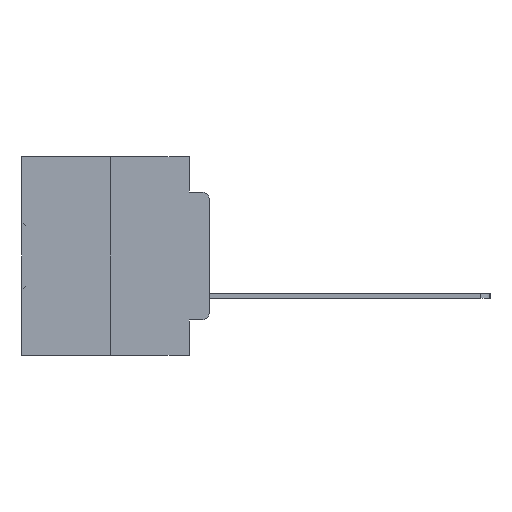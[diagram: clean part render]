
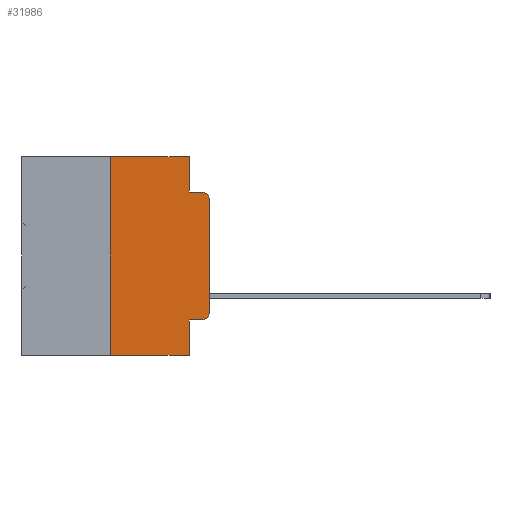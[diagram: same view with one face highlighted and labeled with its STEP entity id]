
A CAD part, left-side view. The second image highlights one B-rep face of the part: STEP entity #31986.
In plain terms, the highlighted planar face has unit normal (-1, 0, 0).
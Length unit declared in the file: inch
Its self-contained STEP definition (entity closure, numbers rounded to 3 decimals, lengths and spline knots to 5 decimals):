
#34 = CARTESIAN_POINT ( 'NONE',  ( 0., 0.051, -0.0885 ) ) ;
#468 = CARTESIAN_POINT ( 'NONE',  ( 0., 0.051, -0.5 ) ) ;
#720 = CARTESIAN_POINT ( 'NONE',  ( 0., 0.051, 0. ) ) ;
#902 = CARTESIAN_POINT ( 'NONE',  ( 0., 0.051, -0.4115 ) ) ;
#982 = CARTESIAN_POINT ( 'NONE',  ( 0., 0., -0.1085 ) ) ;
#1064 = VECTOR ( 'NONE', #9573, 39.37008 ) ;
#1065 = VERTEX_POINT ( 'NONE', #982 ) ;
#1496 = VERTEX_POINT ( 'NONE', #468 ) ;
#1793 = FACE_OUTER_BOUND ( 'NONE', #23797, .T. ) ;
#3012 = EDGE_CURVE ( 'NONE', #28477, #24583, #29889, .T. ) ;
#3042 = AXIS2_PLACEMENT_3D ( 'NONE', #6347, #25291, #9121 ) ;
#3171 = DIRECTION ( 'NONE',  ( 0., 0., 1. ) ) ;
#3943 = VECTOR ( 'NONE', #19839, 39.37008 ) ;
#4041 = DIRECTION ( 'NONE',  ( 0., -1., 0. ) ) ;
#4049 = VECTOR ( 'NONE', #10755, 39.37008 ) ;
#4893 = EDGE_CURVE ( 'NONE', #28477, #1496, #25623, .T. ) ;
#4903 = ORIENTED_EDGE ( 'NONE', *, *, #6758, .F. ) ;
#6218 = ORIENTED_EDGE ( 'NONE', *, *, #30897, .T. ) ;
#6347 = CARTESIAN_POINT ( 'NONE',  ( 0., 0.02, -0.1085 ) ) ;
#6378 = DIRECTION ( 'NONE',  ( -1., 0., 0. ) ) ;
#6604 = CARTESIAN_POINT ( 'NONE',  ( 0., 0.051, -0.0885 ) ) ;
#6731 = CARTESIAN_POINT ( 'NONE',  ( 0., 0.473, 0. ) ) ;
#6758 = EDGE_CURVE ( 'NONE', #26242, #31788, #13685, .T. ) ;
#7073 = VECTOR ( 'NONE', #21686, 39.37008 ) ;
#7951 = CARTESIAN_POINT ( 'NONE',  ( 0., 0.02, -0.4115 ) ) ;
#8803 = CIRCLE ( 'NONE', #24824, 0.02 ) ;
#8840 = LINE ( 'NONE', #6731, #29477 ) ;
#9121 = DIRECTION ( 'NONE',  ( 0., 0., -1. ) ) ;
#9237 = ORIENTED_EDGE ( 'NONE', *, *, #19950, .T. ) ;
#9573 = DIRECTION ( 'NONE',  ( 0., -1., 0. ) ) ;
#9653 = ORIENTED_EDGE ( 'NONE', *, *, #14054, .F. ) ;
#10421 = CARTESIAN_POINT ( 'NONE',  ( 0., 0.051, 0. ) ) ;
#10579 = CARTESIAN_POINT ( 'NONE',  ( 0., 0.25, -0.5 ) ) ;
#10755 = DIRECTION ( 'NONE',  ( 0., -1., 0. ) ) ;
#11082 = DIRECTION ( 'NONE',  ( 1., 0., 0. ) ) ;
#11519 = VERTEX_POINT ( 'NONE', #20777 ) ;
#11705 = DIRECTION ( 'NONE',  ( 0., 0., 1. ) ) ;
#12249 = EDGE_CURVE ( 'NONE', #25033, #15721, #30239, .T. ) ;
#13484 = LINE ( 'NONE', #6604, #18943 ) ;
#13685 = LINE ( 'NONE', #27848, #32511 ) ;
#14054 = EDGE_CURVE ( 'NONE', #15721, #17731, #13484, .T. ) ;
#15134 = ORIENTED_EDGE ( 'NONE', *, *, #15868, .T. ) ;
#15721 = VERTEX_POINT ( 'NONE', #34 ) ;
#15868 = EDGE_CURVE ( 'NONE', #1065, #17731, #16267, .T. ) ;
#16267 = CIRCLE ( 'NONE', #3042, 0.02 ) ;
#17731 = VERTEX_POINT ( 'NONE', #29797 ) ;
#18111 = ORIENTED_EDGE ( 'NONE', *, *, #4893, .F. ) ;
#18943 = VECTOR ( 'NONE', #28223, 39.37008 ) ;
#19476 = EDGE_CURVE ( 'NONE', #11519, #1065, #26607, .T. ) ;
#19839 = DIRECTION ( 'NONE',  ( 0., 0., -1. ) ) ;
#19950 = EDGE_CURVE ( 'NONE', #26242, #1496, #32732, .T. ) ;
#20318 = CARTESIAN_POINT ( 'NONE',  ( 0., 0.051, -0.4115 ) ) ;
#20777 = CARTESIAN_POINT ( 'NONE',  ( 0., 0., -0.3915 ) ) ;
#20922 = CARTESIAN_POINT ( 'NONE',  ( 0., 0.25, 0. ) ) ;
#21392 = CARTESIAN_POINT ( 'NONE',  ( 0., 0.473, -0.5 ) ) ;
#21480 = ORIENTED_EDGE ( 'NONE', *, *, #19476, .T. ) ;
#21686 = DIRECTION ( 'NONE',  ( 0., 0., -1. ) ) ;
#22640 = CARTESIAN_POINT ( 'NONE',  ( 0., 0.02, -0.3915 ) ) ;
#23797 = EDGE_LOOP ( 'NONE', ( #21480, #15134, #9653, #31063, #25699, #4903, #9237, #18111, #32322, #6218 ) ) ;
#24556 = CARTESIAN_POINT ( 'NONE',  ( 0., 0.473, 0. ) ) ;
#24583 = VERTEX_POINT ( 'NONE', #7951 ) ;
#24824 = AXIS2_PLACEMENT_3D ( 'NONE', #22640, #6378, #25323 ) ;
#25033 = VERTEX_POINT ( 'NONE', #10421 ) ;
#25291 = DIRECTION ( 'NONE',  ( -1., 0., 0. ) ) ;
#25323 = DIRECTION ( 'NONE',  ( 0., 0., -1. ) ) ;
#25623 = LINE ( 'NONE', #720, #3943 ) ;
#25699 = ORIENTED_EDGE ( 'NONE', *, *, #32884, .F. ) ;
#26242 = VERTEX_POINT ( 'NONE', #10579 ) ;
#26607 = LINE ( 'NONE', #32791, #33599 ) ;
#27249 = PLANE ( 'NONE',  #29309 ) ;
#27848 = CARTESIAN_POINT ( 'NONE',  ( 0., 0.25, 0. ) ) ;
#28223 = DIRECTION ( 'NONE',  ( 0., -1., 0. ) ) ;
#28477 = VERTEX_POINT ( 'NONE', #902 ) ;
#29309 = AXIS2_PLACEMENT_3D ( 'NONE', #24556, #11082, #29877 ) ;
#29477 = VECTOR ( 'NONE', #4041, 39.37008 ) ;
#29615 = CARTESIAN_POINT ( 'NONE',  ( 0., 0.051, 0. ) ) ;
#29797 = CARTESIAN_POINT ( 'NONE',  ( 0., 0.02, -0.0885 ) ) ;
#29877 = DIRECTION ( 'NONE',  ( 0., 0., -1. ) ) ;
#29889 = LINE ( 'NONE', #20318, #1064 ) ;
#30239 = LINE ( 'NONE', #29615, #7073 ) ;
#30897 = EDGE_CURVE ( 'NONE', #24583, #11519, #8803, .T. ) ;
#31063 = ORIENTED_EDGE ( 'NONE', *, *, #12249, .F. ) ;
#31788 = VERTEX_POINT ( 'NONE', #20922 ) ;
#31986 = ADVANCED_FACE ( 'NONE', ( #1793 ), #27249, .F. ) ;
#32322 = ORIENTED_EDGE ( 'NONE', *, *, #3012, .T. ) ;
#32511 = VECTOR ( 'NONE', #11705, 39.37008 ) ;
#32732 = LINE ( 'NONE', #21392, #4049 ) ;
#32791 = CARTESIAN_POINT ( 'NONE',  ( 0., 0., 0. ) ) ;
#32884 = EDGE_CURVE ( 'NONE', #31788, #25033, #8840, .T. ) ;
#33599 = VECTOR ( 'NONE', #3171, 39.37008 ) ;
